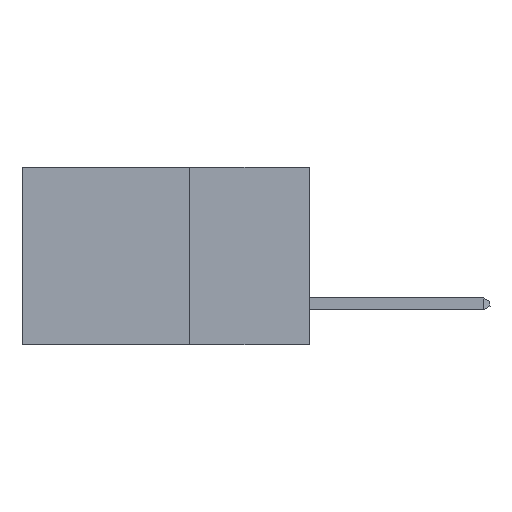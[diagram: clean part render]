
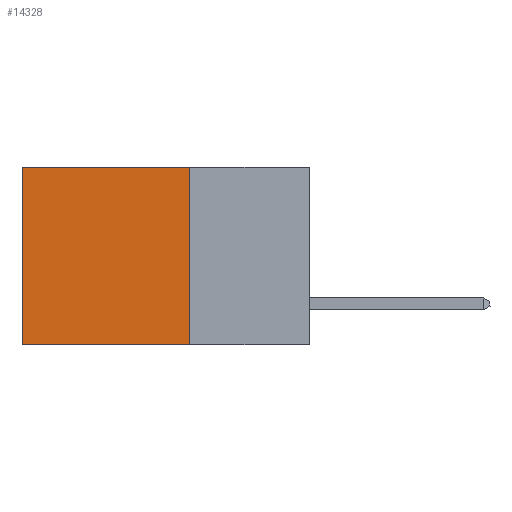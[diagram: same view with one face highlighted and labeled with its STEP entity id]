
A CAD part, left-side view. The second image highlights one B-rep face of the part: STEP entity #14328.
In plain terms, the highlighted planar face has unit normal (-1, 0, 0).
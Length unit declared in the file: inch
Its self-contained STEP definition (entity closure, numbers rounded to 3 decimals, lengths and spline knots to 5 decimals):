
#303 = EDGE_CURVE ( 'NONE', #12608, #19082, #1981, .T. ) ;
#1276 = CARTESIAN_POINT ( 'NONE',  ( 0.2875, 0.25, 0. ) ) ;
#1360 = DIRECTION ( 'NONE',  ( 0., 1., 0. ) ) ;
#1407 = PLANE ( 'NONE',  #18499 ) ;
#1550 = ORIENTED_EDGE ( 'NONE', *, *, #5887, .F. ) ;
#1981 = LINE ( 'NONE', #12159, #20207 ) ;
#2098 = LINE ( 'NONE', #1276, #6262 ) ;
#2922 = VERTEX_POINT ( 'NONE', #21341 ) ;
#3943 = CARTESIAN_POINT ( 'NONE',  ( 0.2875, 0.25, -0.37 ) ) ;
#4344 = FACE_OUTER_BOUND ( 'NONE', #13219, .T. ) ;
#4503 = ORIENTED_EDGE ( 'NONE', *, *, #16760, .T. ) ;
#4679 = VERTEX_POINT ( 'NONE', #20994 ) ;
#4975 = DIRECTION ( 'NONE',  ( 0., 0., -1. ) ) ;
#5569 = ORIENTED_EDGE ( 'NONE', *, *, #12889, .T. ) ;
#5887 = EDGE_CURVE ( 'NONE', #2922, #12608, #10582, .T. ) ;
#5977 = VECTOR ( 'NONE', #10864, 39.37008 ) ;
#6262 = VECTOR ( 'NONE', #1360, 39.37008 ) ;
#6488 = CARTESIAN_POINT ( 'NONE',  ( 0.2875, 0.6, 0. ) ) ;
#9124 = CARTESIAN_POINT ( 'NONE',  ( 0.2875, 0.25, 0. ) ) ;
#10582 = LINE ( 'NONE', #9124, #5977 ) ;
#10656 = DIRECTION ( 'NONE',  ( 0., 1., 0. ) ) ;
#10864 = DIRECTION ( 'NONE',  ( 0., 0., -1. ) ) ;
#11677 = CARTESIAN_POINT ( 'NONE',  ( 0.2875, 0.6, -0.37 ) ) ;
#12159 = CARTESIAN_POINT ( 'NONE',  ( 0.2875, 0.25, -0.37 ) ) ;
#12608 = VERTEX_POINT ( 'NONE', #3943 ) ;
#12824 = LINE ( 'NONE', #6488, #21203 ) ;
#12889 = EDGE_CURVE ( 'NONE', #4679, #19082, #12824, .T. ) ;
#13219 = EDGE_LOOP ( 'NONE', ( #5569, #15097, #1550, #4503 ) ) ;
#13503 = CARTESIAN_POINT ( 'NONE',  ( 0.2875, 0.25, 0. ) ) ;
#14328 = ADVANCED_FACE ( 'NONE', ( #4344 ), #1407, .F. ) ;
#15097 = ORIENTED_EDGE ( 'NONE', *, *, #303, .F. ) ;
#15279 = DIRECTION ( 'NONE',  ( 1., 0., 0. ) ) ;
#16760 = EDGE_CURVE ( 'NONE', #2922, #4679, #2098, .T. ) ;
#18499 = AXIS2_PLACEMENT_3D ( 'NONE', #13503, #15279, #4975 ) ;
#19082 = VERTEX_POINT ( 'NONE', #11677 ) ;
#20207 = VECTOR ( 'NONE', #10656, 39.37008 ) ;
#20994 = CARTESIAN_POINT ( 'NONE',  ( 0.2875, 0.6, 0. ) ) ;
#21203 = VECTOR ( 'NONE', #21742, 39.37008 ) ;
#21341 = CARTESIAN_POINT ( 'NONE',  ( 0.2875, 0.25, 0. ) ) ;
#21742 = DIRECTION ( 'NONE',  ( 0., 0., -1. ) ) ;
